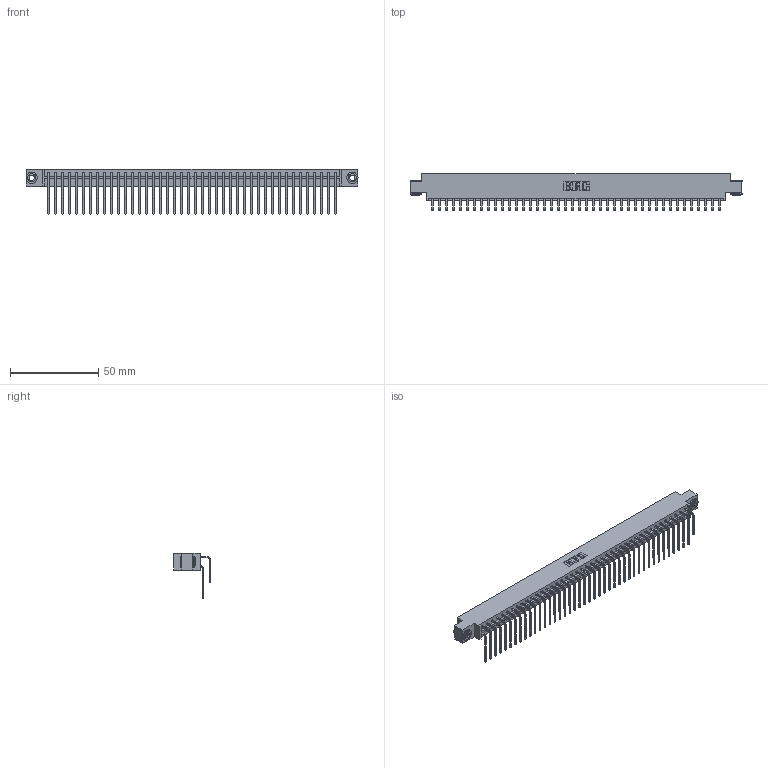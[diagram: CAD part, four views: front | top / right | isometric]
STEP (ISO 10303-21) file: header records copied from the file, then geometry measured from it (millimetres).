
FILE_DESCRIPTION (( 'STEP AP203' ), '1' );
FILE_NAME ('833-084-559-803.STEP', '2020-06-06T02:23:37', ( '' ), ( '' ), 'SwSTEP 2.0', 'SolidWorks 2020', '' );
FILE_SCHEMA (( 'CONFIG_CONTROL_DESIGN' ));
Length unit declared in the file: inch
Products named in the file (5): 345-292-001_559 Tail - 2; 345-292-001_558 559 Tail - 1; 345-250-002_345-250-002-102; 833 Part_Offset - .156 Dia - TH; 833-084-559-803
Assembly tree (87 placements, depth 2):
  833-084-559-803
    833 Part_Offset - .156 Dia - TH
    345-292-001_558 559 Tail - 1  x42
    345-292-001_559 Tail - 2  x42
    345-250-002_345-250-002-102  x2
Bounding box: 187.96 x 20.9 x 25.53 mm (x, y, z)
Volume: 19465.8 mm3; surface area: 25868.8 mm2
Topology: 87 solids, 87 shells, 4692 faces, 13923 edges, 9166 vertices
Faces by surface type: plane 3276, cylinder 1408, cone 8
Entity records: 29586 total; most frequent: CARTESIAN_POINT 4932, ORIENTED_EDGE 4810, DIRECTION 4227, EDGE_CURVE 2405, LINE 2213, VECTOR 2213, VERTEX_POINT 1598, AXIS2_PLACEMENT_3D 1007
